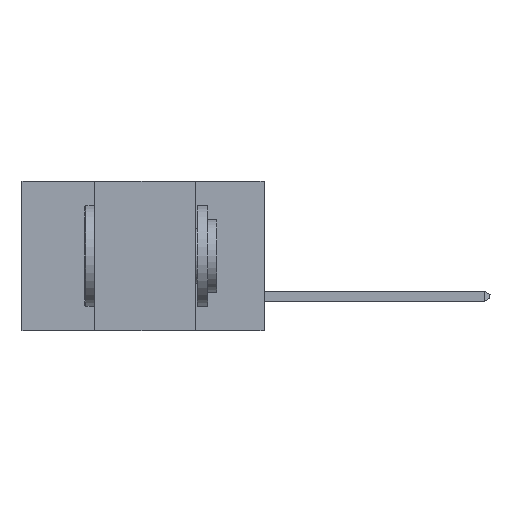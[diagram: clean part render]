
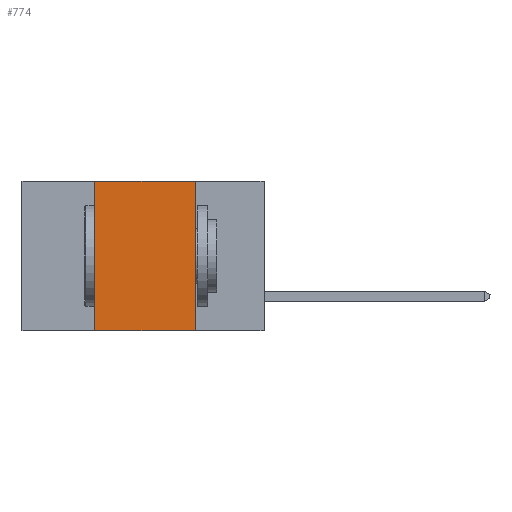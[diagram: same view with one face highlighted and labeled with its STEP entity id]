
A CAD part, left-side view. The second image highlights one B-rep face of the part: STEP entity #774.
In plain terms, the highlighted planar face has unit normal (-1, 0, 0).
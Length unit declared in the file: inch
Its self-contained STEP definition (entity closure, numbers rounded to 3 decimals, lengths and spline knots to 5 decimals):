
#570 = ORIENTED_EDGE ( 'NONE', *, *, #10059, .T. ) ;
#774 = ADVANCED_FACE ( 'NONE', ( #4355 ), #5934, .F. ) ;
#1061 = DIRECTION ( 'NONE',  ( 0., 0., 1. ) ) ;
#1569 = DIRECTION ( 'NONE',  ( 1., 0., 0. ) ) ;
#1703 = CARTESIAN_POINT ( 'NONE',  ( 0., 0.42, 0. ) ) ;
#1762 = CARTESIAN_POINT ( 'NONE',  ( 0., 0.6, -0.37 ) ) ;
#2039 = VERTEX_POINT ( 'NONE', #10203 ) ;
#2429 = DIRECTION ( 'NONE',  ( 0., 0., -1. ) ) ;
#2456 = DIRECTION ( 'NONE',  ( 0., 0., -1. ) ) ;
#2583 = DIRECTION ( 'NONE',  ( 0., -1., 0. ) ) ;
#2651 = VECTOR ( 'NONE', #1061, 39.37008 ) ;
#2676 = CARTESIAN_POINT ( 'NONE',  ( 0., 0.6, 0. ) ) ;
#3661 = VECTOR ( 'NONE', #2583, 39.37008 ) ;
#3754 = VECTOR ( 'NONE', #2456, 39.37008 ) ;
#3902 = ORIENTED_EDGE ( 'NONE', *, *, #9336, .F. ) ;
#4134 = CARTESIAN_POINT ( 'NONE',  ( 0., 0.17, 0. ) ) ;
#4280 = CARTESIAN_POINT ( 'NONE',  ( 0., 0.42, -0.37 ) ) ;
#4355 = FACE_OUTER_BOUND ( 'NONE', #5933, .T. ) ;
#4734 = VERTEX_POINT ( 'NONE', #1703 ) ;
#5046 = ORIENTED_EDGE ( 'NONE', *, *, #5770, .F. ) ;
#5770 = EDGE_CURVE ( 'NONE', #10230, #2039, #7103, .T. ) ;
#5933 = EDGE_LOOP ( 'NONE', ( #5046, #10484, #3902, #570 ) ) ;
#5934 = PLANE ( 'NONE',  #6962 ) ;
#6962 = AXIS2_PLACEMENT_3D ( 'NONE', #2676, #1569, #2429 ) ;
#7103 = LINE ( 'NONE', #4134, #3754 ) ;
#7207 = CARTESIAN_POINT ( 'NONE',  ( 0., 0.17, 0. ) ) ;
#7860 = DIRECTION ( 'NONE',  ( 0., -1., 0. ) ) ;
#8532 = LINE ( 'NONE', #9973, #2651 ) ;
#9024 = LINE ( 'NONE', #10238, #9150 ) ;
#9150 = VECTOR ( 'NONE', #7860, 39.37008 ) ;
#9336 = EDGE_CURVE ( 'NONE', #9838, #4734, #8532, .T. ) ;
#9778 = EDGE_CURVE ( 'NONE', #4734, #10230, #9024, .T. ) ;
#9838 = VERTEX_POINT ( 'NONE', #4280 ) ;
#9973 = CARTESIAN_POINT ( 'NONE',  ( 0., 0.42, 0. ) ) ;
#10029 = LINE ( 'NONE', #1762, #3661 ) ;
#10059 = EDGE_CURVE ( 'NONE', #9838, #2039, #10029, .T. ) ;
#10203 = CARTESIAN_POINT ( 'NONE',  ( 0., 0.17, -0.37 ) ) ;
#10230 = VERTEX_POINT ( 'NONE', #7207 ) ;
#10238 = CARTESIAN_POINT ( 'NONE',  ( 0., 0.6, 0. ) ) ;
#10484 = ORIENTED_EDGE ( 'NONE', *, *, #9778, .F. ) ;
